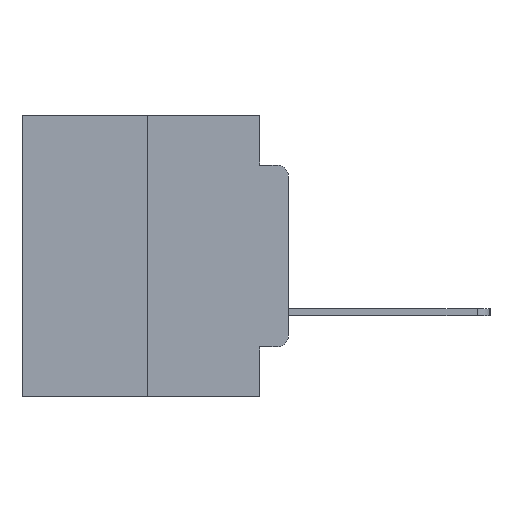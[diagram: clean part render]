
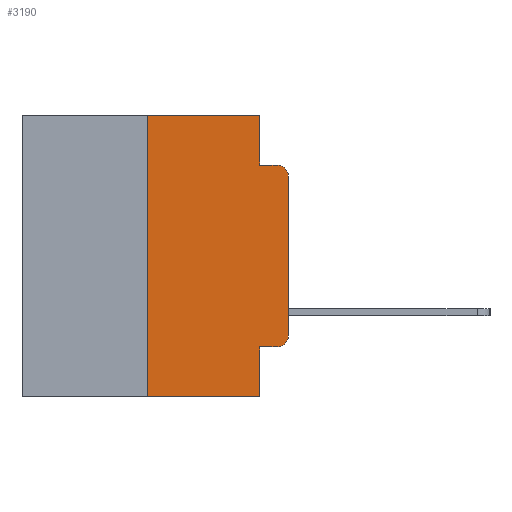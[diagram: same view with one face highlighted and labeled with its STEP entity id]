
A CAD part, left-side view. The second image highlights one B-rep face of the part: STEP entity #3190.
In plain terms, the highlighted planar face has unit normal (-1, 0, 0).
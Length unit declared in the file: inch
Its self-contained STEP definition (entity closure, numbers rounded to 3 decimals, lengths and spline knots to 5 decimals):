
#118 = EDGE_CURVE ( 'NONE', #10177, #20772, #1781, .T. ) ;
#247 = DIRECTION ( 'NONE',  ( 0., -1., 0. ) ) ;
#1307 = VECTOR ( 'NONE', #17497, 39.37008 ) ;
#1781 = LINE ( 'NONE', #4811, #17112 ) ;
#1989 = CARTESIAN_POINT ( 'NONE',  ( 0., 0., 0. ) ) ;
#2369 = EDGE_CURVE ( 'NONE', #14720, #23418, #13435, .T. ) ;
#2375 = LINE ( 'NONE', #9032, #12554 ) ;
#3011 = EDGE_CURVE ( 'NONE', #23145, #20772, #2375, .T. ) ;
#3190 = ADVANCED_FACE ( 'NONE', ( #23499 ), #8028, .F. ) ;
#3615 = VECTOR ( 'NONE', #22100, 39.37008 ) ;
#4115 = LINE ( 'NONE', #23853, #14160 ) ;
#4326 = ORIENTED_EDGE ( 'NONE', *, *, #20194, .F. ) ;
#4414 = EDGE_CURVE ( 'NONE', #23145, #14720, #12157, .T. ) ;
#4811 = CARTESIAN_POINT ( 'NONE',  ( 0., 0.051, 0. ) ) ;
#4936 = VERTEX_POINT ( 'NONE', #23929 ) ;
#4943 = CARTESIAN_POINT ( 'NONE',  ( 0., 0.051, -0.4115 ) ) ;
#5030 = VERTEX_POINT ( 'NONE', #11261 ) ;
#5632 = ORIENTED_EDGE ( 'NONE', *, *, #4414, .F. ) ;
#5928 = EDGE_LOOP ( 'NONE', ( #11307, #17587, #4326, #14924, #20567, #5632, #11617, #23473, #24047, #20296 ) ) ;
#6621 = VERTEX_POINT ( 'NONE', #13209 ) ;
#6896 = VECTOR ( 'NONE', #23432, 39.37008 ) ;
#7548 = LINE ( 'NONE', #1989, #17271 ) ;
#8028 = PLANE ( 'NONE',  #17671 ) ;
#8160 = LINE ( 'NONE', #15400, #22842 ) ;
#8709 = CARTESIAN_POINT ( 'NONE',  ( 0., 0.051, 0. ) ) ;
#9032 = CARTESIAN_POINT ( 'NONE',  ( 0., 0.473, -0.5 ) ) ;
#9818 = CARTESIAN_POINT ( 'NONE',  ( 0., 0.473, 0. ) ) ;
#9838 = CARTESIAN_POINT ( 'NONE',  ( 0., 0.473, 0. ) ) ;
#9916 = EDGE_CURVE ( 'NONE', #23418, #4936, #13712, .T. ) ;
#10172 = CARTESIAN_POINT ( 'NONE',  ( 0., 0.051, -0.5 ) ) ;
#10177 = VERTEX_POINT ( 'NONE', #4943 ) ;
#10948 = DIRECTION ( 'NONE',  ( -1., 0., 0. ) ) ;
#11261 = CARTESIAN_POINT ( 'NONE',  ( 0., 0., -0.3915 ) ) ;
#11307 = ORIENTED_EDGE ( 'NONE', *, *, #23901, .T. ) ;
#11341 = CARTESIAN_POINT ( 'NONE',  ( 0., 0.02, -0.3915 ) ) ;
#11387 = CARTESIAN_POINT ( 'NONE',  ( 0., 0.25, 0. ) ) ;
#11617 = ORIENTED_EDGE ( 'NONE', *, *, #3011, .T. ) ;
#11771 = VERTEX_POINT ( 'NONE', #23822 ) ;
#11865 = CARTESIAN_POINT ( 'NONE',  ( 0., 0.25, -0.5 ) ) ;
#11960 = CIRCLE ( 'NONE', #24393, 0.02 ) ;
#11996 = DIRECTION ( 'NONE',  ( 1., 0., 0. ) ) ;
#12157 = LINE ( 'NONE', #15049, #6896 ) ;
#12450 = CARTESIAN_POINT ( 'NONE',  ( 0., 0.02, -0.0885 ) ) ;
#12554 = VECTOR ( 'NONE', #18284, 39.37008 ) ;
#13209 = CARTESIAN_POINT ( 'NONE',  ( 0., 0., -0.1085 ) ) ;
#13279 = DIRECTION ( 'NONE',  ( 0., 0., -1. ) ) ;
#13435 = LINE ( 'NONE', #9818, #1307 ) ;
#13712 = LINE ( 'NONE', #8709, #3615 ) ;
#14160 = VECTOR ( 'NONE', #247, 39.37008 ) ;
#14720 = VERTEX_POINT ( 'NONE', #11387 ) ;
#14924 = ORIENTED_EDGE ( 'NONE', *, *, #9916, .F. ) ;
#15049 = CARTESIAN_POINT ( 'NONE',  ( 0., 0.25, 0. ) ) ;
#15400 = CARTESIAN_POINT ( 'NONE',  ( 0., 0.051, -0.4115 ) ) ;
#17112 = VECTOR ( 'NONE', #18153, 39.37008 ) ;
#17271 = VECTOR ( 'NONE', #19873, 39.37008 ) ;
#17322 = DIRECTION ( 'NONE',  ( 0., -1., 0. ) ) ;
#17484 = AXIS2_PLACEMENT_3D ( 'NONE', #11341, #24545, #13279 ) ;
#17497 = DIRECTION ( 'NONE',  ( 0., -1., 0. ) ) ;
#17587 = ORIENTED_EDGE ( 'NONE', *, *, #21444, .T. ) ;
#17671 = AXIS2_PLACEMENT_3D ( 'NONE', #9838, #11996, #23348 ) ;
#18153 = DIRECTION ( 'NONE',  ( 0., 0., -1. ) ) ;
#18284 = DIRECTION ( 'NONE',  ( 0., -1., 0. ) ) ;
#19378 = EDGE_CURVE ( 'NONE', #11771, #5030, #21473, .T. ) ;
#19873 = DIRECTION ( 'NONE',  ( 0., 0., 1. ) ) ;
#20194 = EDGE_CURVE ( 'NONE', #4936, #23356, #4115, .T. ) ;
#20296 = ORIENTED_EDGE ( 'NONE', *, *, #19378, .T. ) ;
#20567 = ORIENTED_EDGE ( 'NONE', *, *, #2369, .F. ) ;
#20772 = VERTEX_POINT ( 'NONE', #10172 ) ;
#21444 = EDGE_CURVE ( 'NONE', #6621, #23356, #11960, .T. ) ;
#21473 = CIRCLE ( 'NONE', #17484, 0.02 ) ;
#22100 = DIRECTION ( 'NONE',  ( 0., 0., -1. ) ) ;
#22320 = CARTESIAN_POINT ( 'NONE',  ( 0., 0.02, -0.1085 ) ) ;
#22842 = VECTOR ( 'NONE', #17322, 39.37008 ) ;
#23145 = VERTEX_POINT ( 'NONE', #11865 ) ;
#23348 = DIRECTION ( 'NONE',  ( 0., 0., -1. ) ) ;
#23356 = VERTEX_POINT ( 'NONE', #12450 ) ;
#23418 = VERTEX_POINT ( 'NONE', #24007 ) ;
#23432 = DIRECTION ( 'NONE',  ( 0., 0., 1. ) ) ;
#23473 = ORIENTED_EDGE ( 'NONE', *, *, #118, .F. ) ;
#23499 = FACE_OUTER_BOUND ( 'NONE', #5928, .T. ) ;
#23822 = CARTESIAN_POINT ( 'NONE',  ( 0., 0.02, -0.4115 ) ) ;
#23853 = CARTESIAN_POINT ( 'NONE',  ( 0., 0.051, -0.0885 ) ) ;
#23901 = EDGE_CURVE ( 'NONE', #5030, #6621, #7548, .T. ) ;
#23929 = CARTESIAN_POINT ( 'NONE',  ( 0., 0.051, -0.0885 ) ) ;
#24007 = CARTESIAN_POINT ( 'NONE',  ( 0., 0.051, 0. ) ) ;
#24047 = ORIENTED_EDGE ( 'NONE', *, *, #24346, .T. ) ;
#24163 = DIRECTION ( 'NONE',  ( 0., 0., -1. ) ) ;
#24346 = EDGE_CURVE ( 'NONE', #10177, #11771, #8160, .T. ) ;
#24393 = AXIS2_PLACEMENT_3D ( 'NONE', #22320, #10948, #24163 ) ;
#24545 = DIRECTION ( 'NONE',  ( -1., 0., 0. ) ) ;
